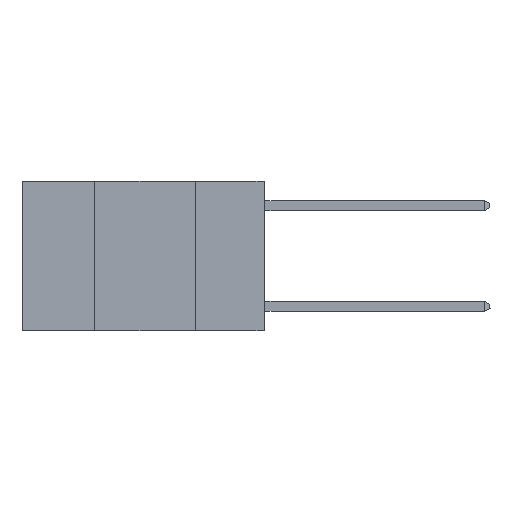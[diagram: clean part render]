
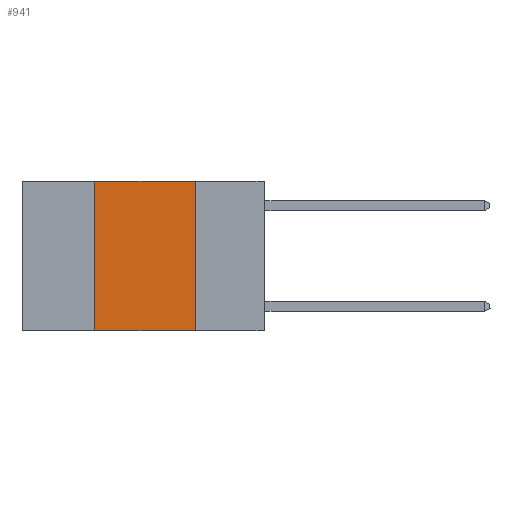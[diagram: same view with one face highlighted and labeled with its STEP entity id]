
A CAD part, left-side view. The second image highlights one B-rep face of the part: STEP entity #941.
In plain terms, the highlighted planar face has unit normal (-1, 0, 0).
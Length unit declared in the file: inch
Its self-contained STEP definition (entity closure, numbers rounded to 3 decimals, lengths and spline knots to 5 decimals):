
#108 = DIRECTION ( 'NONE',  ( 1., 0., 0. ) ) ;
#141 = LINE ( 'NONE', #8133, #6783 ) ;
#334 = LINE ( 'NONE', #4756, #2765 ) ;
#353 = CARTESIAN_POINT ( 'NONE',  ( 0., 0.6, -0.37 ) ) ;
#583 = VERTEX_POINT ( 'NONE', #3929 ) ;
#645 = EDGE_CURVE ( 'NONE', #583, #7591, #334, .T. ) ;
#723 = CARTESIAN_POINT ( 'NONE',  ( 0., 0.42, 0. ) ) ;
#941 = ADVANCED_FACE ( 'NONE', ( #4909 ), #7516, .F. ) ;
#1361 = ORIENTED_EDGE ( 'NONE', *, *, #645, .F. ) ;
#1637 = CARTESIAN_POINT ( 'NONE',  ( 0., 0.6, 0. ) ) ;
#1773 = DIRECTION ( 'NONE',  ( 0., -1., 0. ) ) ;
#1815 = ORIENTED_EDGE ( 'NONE', *, *, #3854, .F. ) ;
#1913 = ORIENTED_EDGE ( 'NONE', *, *, #7766, .F. ) ;
#2008 = VERTEX_POINT ( 'NONE', #723 ) ;
#2252 = CARTESIAN_POINT ( 'NONE',  ( 0., 0.17, -0.37 ) ) ;
#2274 = DIRECTION ( 'NONE',  ( 0., 0., 1. ) ) ;
#2765 = VECTOR ( 'NONE', #6776, 39.37008 ) ;
#3785 = CARTESIAN_POINT ( 'NONE',  ( 0., 0.6, 0. ) ) ;
#3854 = EDGE_CURVE ( 'NONE', #6942, #2008, #141, .T. ) ;
#3929 = CARTESIAN_POINT ( 'NONE',  ( 0., 0.17, 0. ) ) ;
#3973 = EDGE_CURVE ( 'NONE', #6942, #7591, #6241, .T. ) ;
#4055 = VECTOR ( 'NONE', #5612, 39.37008 ) ;
#4756 = CARTESIAN_POINT ( 'NONE',  ( 0., 0.17, 0. ) ) ;
#4909 = FACE_OUTER_BOUND ( 'NONE', #5767, .T. ) ;
#5381 = DIRECTION ( 'NONE',  ( 0., 0., -1. ) ) ;
#5612 = DIRECTION ( 'NONE',  ( 0., -1., 0. ) ) ;
#5656 = AXIS2_PLACEMENT_3D ( 'NONE', #1637, #108, #5381 ) ;
#5701 = CARTESIAN_POINT ( 'NONE',  ( 0., 0.42, -0.37 ) ) ;
#5767 = EDGE_LOOP ( 'NONE', ( #1361, #1913, #1815, #7193 ) ) ;
#6241 = LINE ( 'NONE', #353, #4055 ) ;
#6776 = DIRECTION ( 'NONE',  ( 0., 0., -1. ) ) ;
#6783 = VECTOR ( 'NONE', #2274, 39.37008 ) ;
#6942 = VERTEX_POINT ( 'NONE', #5701 ) ;
#7193 = ORIENTED_EDGE ( 'NONE', *, *, #3973, .T. ) ;
#7516 = PLANE ( 'NONE',  #5656 ) ;
#7591 = VERTEX_POINT ( 'NONE', #2252 ) ;
#7674 = LINE ( 'NONE', #3785, #8289 ) ;
#7766 = EDGE_CURVE ( 'NONE', #2008, #583, #7674, .T. ) ;
#8133 = CARTESIAN_POINT ( 'NONE',  ( 0., 0.42, 0. ) ) ;
#8289 = VECTOR ( 'NONE', #1773, 39.37008 ) ;
